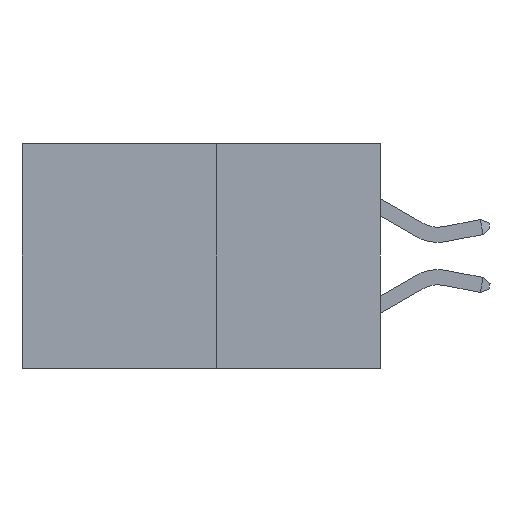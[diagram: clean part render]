
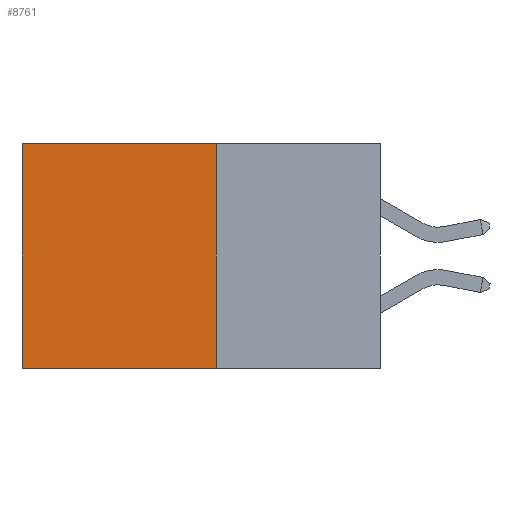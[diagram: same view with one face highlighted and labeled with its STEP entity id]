
A CAD part, left-side view. The second image highlights one B-rep face of the part: STEP entity #8761.
In plain terms, the highlighted planar face has unit normal (-1, 0, 0).
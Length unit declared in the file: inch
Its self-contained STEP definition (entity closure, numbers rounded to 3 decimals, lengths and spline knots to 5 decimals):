
#707 = VERTEX_POINT ( 'NONE', #8770 ) ;
#1656 = CARTESIAN_POINT ( 'NONE',  ( 0.277, 0.27, -0.37 ) ) ;
#2029 = VECTOR ( 'NONE', #6690, 39.37008 ) ;
#2303 = VERTEX_POINT ( 'NONE', #4705 ) ;
#2411 = LINE ( 'NONE', #5575, #2029 ) ;
#2841 = VERTEX_POINT ( 'NONE', #7519 ) ;
#3119 = VECTOR ( 'NONE', #13612, 39.37008 ) ;
#3473 = CARTESIAN_POINT ( 'NONE',  ( 0.277, 0.27, 0. ) ) ;
#4092 = EDGE_CURVE ( 'NONE', #707, #2841, #6716, .T. ) ;
#4150 = CARTESIAN_POINT ( 'NONE',  ( 0.277, 0.59, -0.37 ) ) ;
#4520 = DIRECTION ( 'NONE',  ( 0., 0., -1. ) ) ;
#4705 = CARTESIAN_POINT ( 'NONE',  ( 0.277, 0.59, 0. ) ) ;
#4825 = EDGE_CURVE ( 'NONE', #2303, #2841, #11323, .T. ) ;
#5575 = CARTESIAN_POINT ( 'NONE',  ( 0.277, 0.27, -0.37 ) ) ;
#6059 = LINE ( 'NONE', #3473, #3119 ) ;
#6690 = DIRECTION ( 'NONE',  ( 0., 0., -1. ) ) ;
#6716 = LINE ( 'NONE', #1656, #12438 ) ;
#7519 = CARTESIAN_POINT ( 'NONE',  ( 0.277, 0.59, -0.37 ) ) ;
#7580 = AXIS2_PLACEMENT_3D ( 'NONE', #10169, #9659, #9657 ) ;
#8412 = CARTESIAN_POINT ( 'NONE',  ( 0.277, 0.27, 0. ) ) ;
#8521 = EDGE_CURVE ( 'NONE', #11681, #2303, #6059, .T. ) ;
#8761 = ADVANCED_FACE ( 'NONE', ( #14075 ), #9413, .F. ) ;
#8770 = CARTESIAN_POINT ( 'NONE',  ( 0.277, 0.27, -0.37 ) ) ;
#9167 = DIRECTION ( 'NONE',  ( 0., 1., 0. ) ) ;
#9413 = PLANE ( 'NONE',  #7580 ) ;
#9657 = DIRECTION ( 'NONE',  ( 0., 0., -1. ) ) ;
#9659 = DIRECTION ( 'NONE',  ( 1., 0., 0. ) ) ;
#10169 = CARTESIAN_POINT ( 'NONE',  ( 0.277, 0.27, -0.37 ) ) ;
#10282 = ORIENTED_EDGE ( 'NONE', *, *, #8521, .T. ) ;
#11323 = LINE ( 'NONE', #4150, #13398 ) ;
#11681 = VERTEX_POINT ( 'NONE', #8412 ) ;
#12274 = ORIENTED_EDGE ( 'NONE', *, *, #4825, .T. ) ;
#12370 = ORIENTED_EDGE ( 'NONE', *, *, #4092, .F. ) ;
#12438 = VECTOR ( 'NONE', #9167, 39.37008 ) ;
#12693 = ORIENTED_EDGE ( 'NONE', *, *, #13519, .F. ) ;
#13398 = VECTOR ( 'NONE', #4520, 39.37008 ) ;
#13414 = EDGE_LOOP ( 'NONE', ( #12274, #12370, #12693, #10282 ) ) ;
#13519 = EDGE_CURVE ( 'NONE', #11681, #707, #2411, .T. ) ;
#13612 = DIRECTION ( 'NONE',  ( 0., 1., 0. ) ) ;
#14075 = FACE_OUTER_BOUND ( 'NONE', #13414, .T. ) ;
